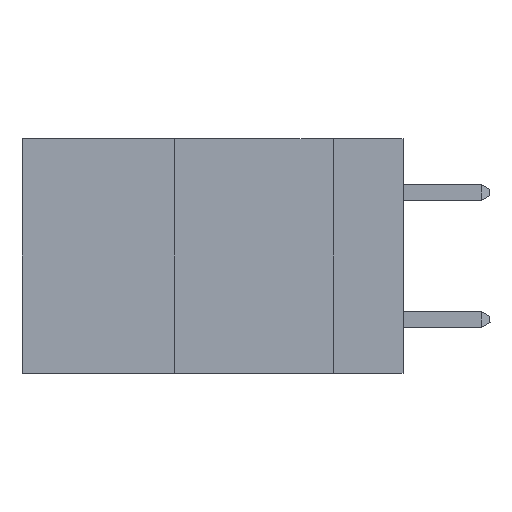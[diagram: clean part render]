
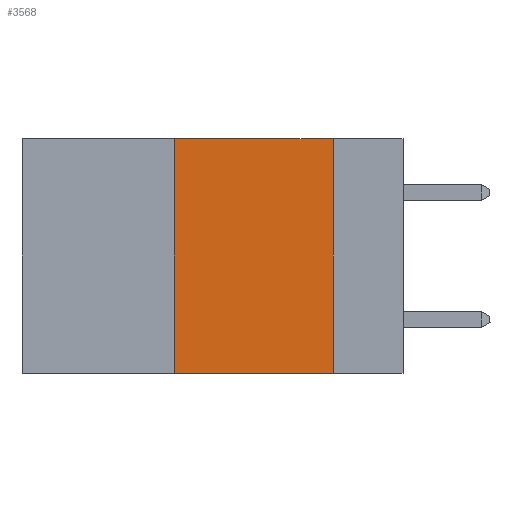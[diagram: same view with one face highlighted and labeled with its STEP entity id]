
A CAD part, left-side view. The second image highlights one B-rep face of the part: STEP entity #3568.
In plain terms, the highlighted planar face has unit normal (-1, 0, 0).
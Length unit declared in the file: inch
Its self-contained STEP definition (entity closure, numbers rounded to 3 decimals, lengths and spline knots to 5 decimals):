
#733 = DIRECTION ( 'NONE',  ( 0., -1., 0. ) ) ;
#1582 = ORIENTED_EDGE ( 'NONE', *, *, #13982, .F. ) ;
#1719 = EDGE_CURVE ( 'NONE', #19904, #1980, #7790, .T. ) ;
#1980 = VERTEX_POINT ( 'NONE', #3114 ) ;
#3114 = CARTESIAN_POINT ( 'NONE',  ( 0., 0.11, 0. ) ) ;
#3568 = ADVANCED_FACE ( 'NONE', ( #6227 ), #10847, .F. ) ;
#4121 = VECTOR ( 'NONE', #18016, 39.37008 ) ;
#4348 = CARTESIAN_POINT ( 'NONE',  ( 0., 0.36, -0.37 ) ) ;
#4531 = CARTESIAN_POINT ( 'NONE',  ( 0., 0.6, 0. ) ) ;
#5503 = CARTESIAN_POINT ( 'NONE',  ( 0., 0.6, 0. ) ) ;
#5905 = CARTESIAN_POINT ( 'NONE',  ( 0., 0.6, -0.37 ) ) ;
#6227 = FACE_OUTER_BOUND ( 'NONE', #8353, .T. ) ;
#7055 = ORIENTED_EDGE ( 'NONE', *, *, #19590, .F. ) ;
#7406 = LINE ( 'NONE', #9449, #11016 ) ;
#7790 = LINE ( 'NONE', #5503, #20862 ) ;
#8353 = EDGE_LOOP ( 'NONE', ( #7055, #17240, #1582, #14072 ) ) ;
#8823 = VERTEX_POINT ( 'NONE', #10846 ) ;
#8962 = LINE ( 'NONE', #5905, #4121 ) ;
#9449 = CARTESIAN_POINT ( 'NONE',  ( 0., 0.11, 0. ) ) ;
#10204 = CARTESIAN_POINT ( 'NONE',  ( 0., 0.36, 0. ) ) ;
#10625 = DIRECTION ( 'NONE',  ( 1., 0., 0. ) ) ;
#10846 = CARTESIAN_POINT ( 'NONE',  ( 0., 0.11, -0.37 ) ) ;
#10847 = PLANE ( 'NONE',  #15210 ) ;
#11016 = VECTOR ( 'NONE', #19596, 39.37008 ) ;
#11076 = DIRECTION ( 'NONE',  ( 0., 0., -1. ) ) ;
#11114 = VECTOR ( 'NONE', #21396, 39.37008 ) ;
#11318 = CARTESIAN_POINT ( 'NONE',  ( 0., 0.36, 0. ) ) ;
#12630 = VERTEX_POINT ( 'NONE', #4348 ) ;
#13982 = EDGE_CURVE ( 'NONE', #12630, #19904, #20094, .T. ) ;
#14072 = ORIENTED_EDGE ( 'NONE', *, *, #17211, .T. ) ;
#15210 = AXIS2_PLACEMENT_3D ( 'NONE', #4531, #10625, #11076 ) ;
#17211 = EDGE_CURVE ( 'NONE', #12630, #8823, #8962, .T. ) ;
#17240 = ORIENTED_EDGE ( 'NONE', *, *, #1719, .F. ) ;
#18016 = DIRECTION ( 'NONE',  ( 0., -1., 0. ) ) ;
#19590 = EDGE_CURVE ( 'NONE', #1980, #8823, #7406, .T. ) ;
#19596 = DIRECTION ( 'NONE',  ( 0., 0., -1. ) ) ;
#19904 = VERTEX_POINT ( 'NONE', #10204 ) ;
#20094 = LINE ( 'NONE', #11318, #11114 ) ;
#20862 = VECTOR ( 'NONE', #733, 39.37008 ) ;
#21396 = DIRECTION ( 'NONE',  ( 0., 0., 1. ) ) ;
